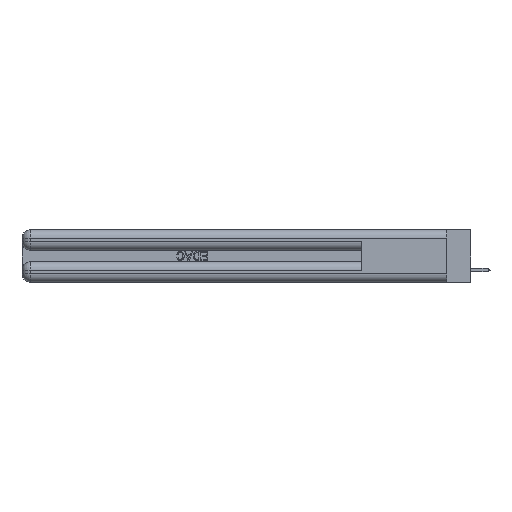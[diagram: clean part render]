
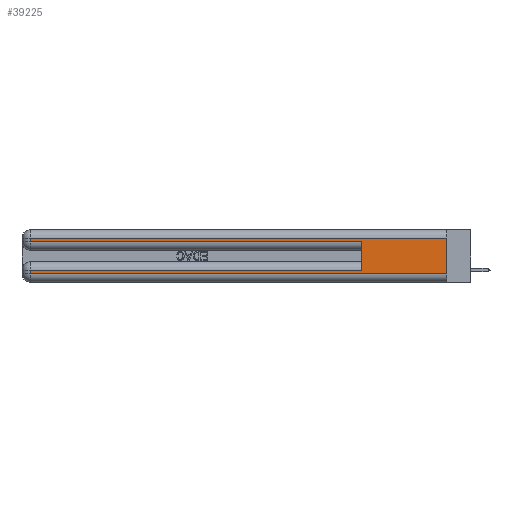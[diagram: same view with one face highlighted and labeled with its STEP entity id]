
A CAD part, left-side view. The second image highlights one B-rep face of the part: STEP entity #39225.
In plain terms, the highlighted planar face has unit normal (-1, 0, 0).
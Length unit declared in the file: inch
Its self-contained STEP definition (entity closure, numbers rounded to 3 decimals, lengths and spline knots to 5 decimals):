
#1727 = EDGE_CURVE ( 'NONE', #25122, #8568, #16309, .T. ) ;
#2623 = DIRECTION ( 'NONE',  ( 1., 0., 0. ) ) ;
#2973 = EDGE_CURVE ( 'NONE', #25122, #19299, #24184, .T. ) ;
#5003 = EDGE_CURVE ( 'NONE', #19886, #38304, #19402, .T. ) ;
#5117 = DIRECTION ( 'NONE',  ( 0., 0., -1. ) ) ;
#5318 = VECTOR ( 'NONE', #33251, 39.37008 ) ;
#7561 = LINE ( 'NONE', #8509, #25066 ) ;
#8483 = DIRECTION ( 'NONE',  ( 0., -1., 0. ) ) ;
#8509 = CARTESIAN_POINT ( 'NONE',  ( 0., 0., 0.37 ) ) ;
#8568 = VERTEX_POINT ( 'NONE', #21581 ) ;
#8902 = DIRECTION ( 'NONE',  ( 0., 0., -1. ) ) ;
#9359 = AXIS2_PLACEMENT_3D ( 'NONE', #15032, #2623, #5117 ) ;
#10208 = VECTOR ( 'NONE', #35673, 39.37008 ) ;
#10851 = CARTESIAN_POINT ( 'NONE',  ( 0., 2.94, 0.085 ) ) ;
#12128 = FACE_OUTER_BOUND ( 'NONE', #35505, .T. ) ;
#14109 = CARTESIAN_POINT ( 'NONE',  ( 0., 2.94, 0.37 ) ) ;
#14813 = LINE ( 'NONE', #34267, #28767 ) ;
#15032 = CARTESIAN_POINT ( 'NONE',  ( 0., 0., 0.37 ) ) ;
#16056 = ORIENTED_EDGE ( 'NONE', *, *, #5003, .T. ) ;
#16309 = LINE ( 'NONE', #19903, #5318 ) ;
#16492 = ORIENTED_EDGE ( 'NONE', *, *, #1727, .F. ) ;
#16751 = EDGE_CURVE ( 'NONE', #26537, #8568, #14813, .T. ) ;
#17328 = ORIENTED_EDGE ( 'NONE', *, *, #19534, .T. ) ;
#18026 = VERTEX_POINT ( 'NONE', #38992 ) ;
#18718 = ORIENTED_EDGE ( 'NONE', *, *, #16751, .T. ) ;
#19065 = LINE ( 'NONE', #14109, #24553 ) ;
#19246 = LINE ( 'NONE', #40370, #41201 ) ;
#19299 = VERTEX_POINT ( 'NONE', #10851 ) ;
#19402 = LINE ( 'NONE', #31055, #39340 ) ;
#19534 = EDGE_CURVE ( 'NONE', #25641, #26537, #19065, .T. ) ;
#19717 = DIRECTION ( 'NONE',  ( 0., 0., -1. ) ) ;
#19886 = VERTEX_POINT ( 'NONE', #36604 ) ;
#19903 = CARTESIAN_POINT ( 'NONE',  ( 0., 0.6, 0.145 ) ) ;
#20246 = DIRECTION ( 'NONE',  ( 0., 0., -1. ) ) ;
#21581 = CARTESIAN_POINT ( 'NONE',  ( 0., 0.6, 0.285 ) ) ;
#22746 = DIRECTION ( 'NONE',  ( 0., 1., 0. ) ) ;
#23398 = ORIENTED_EDGE ( 'NONE', *, *, #23899, .F. ) ;
#23899 = EDGE_CURVE ( 'NONE', #18026, #38304, #7561, .T. ) ;
#24184 = LINE ( 'NONE', #35378, #34629 ) ;
#24553 = VECTOR ( 'NONE', #20246, 39.37008 ) ;
#24842 = DIRECTION ( 'NONE',  ( 0., -1., 0. ) ) ;
#25066 = VECTOR ( 'NONE', #19717, 39.37008 ) ;
#25122 = VERTEX_POINT ( 'NONE', #35357 ) ;
#25641 = VERTEX_POINT ( 'NONE', #28639 ) ;
#26537 = VERTEX_POINT ( 'NONE', #27034 ) ;
#27034 = CARTESIAN_POINT ( 'NONE',  ( 0., 2.94, 0.285 ) ) ;
#28271 = LINE ( 'NONE', #35813, #10208 ) ;
#28639 = CARTESIAN_POINT ( 'NONE',  ( 0., 2.94, 0.31 ) ) ;
#28767 = VECTOR ( 'NONE', #24842, 39.37008 ) ;
#31055 = CARTESIAN_POINT ( 'NONE',  ( 0., 0., 0.06 ) ) ;
#32611 = CARTESIAN_POINT ( 'NONE',  ( 0., 0., 0.06 ) ) ;
#33251 = DIRECTION ( 'NONE',  ( 0., 0., 1. ) ) ;
#33953 = PLANE ( 'NONE',  #9359 ) ;
#34267 = CARTESIAN_POINT ( 'NONE',  ( 0., 0., 0.285 ) ) ;
#34629 = VECTOR ( 'NONE', #22746, 39.37008 ) ;
#34935 = EDGE_CURVE ( 'NONE', #18026, #25641, #28271, .T. ) ;
#35357 = CARTESIAN_POINT ( 'NONE',  ( 0., 0.6, 0.085 ) ) ;
#35378 = CARTESIAN_POINT ( 'NONE',  ( 0., 0., 0.085 ) ) ;
#35446 = ORIENTED_EDGE ( 'NONE', *, *, #34935, .T. ) ;
#35505 = EDGE_LOOP ( 'NONE', ( #23398, #35446, #17328, #18718, #16492, #40643, #36920, #16056 ) ) ;
#35673 = DIRECTION ( 'NONE',  ( 0., 1., 0. ) ) ;
#35813 = CARTESIAN_POINT ( 'NONE',  ( 0., 0., 0.31 ) ) ;
#36443 = EDGE_CURVE ( 'NONE', #19299, #19886, #19246, .T. ) ;
#36604 = CARTESIAN_POINT ( 'NONE',  ( 0., 2.94, 0.06 ) ) ;
#36920 = ORIENTED_EDGE ( 'NONE', *, *, #36443, .T. ) ;
#38304 = VERTEX_POINT ( 'NONE', #32611 ) ;
#38992 = CARTESIAN_POINT ( 'NONE',  ( 0., 0., 0.31 ) ) ;
#39225 = ADVANCED_FACE ( 'NONE', ( #12128 ), #33953, .F. ) ;
#39340 = VECTOR ( 'NONE', #8483, 39.37008 ) ;
#40370 = CARTESIAN_POINT ( 'NONE',  ( 0., 2.94, 0.37 ) ) ;
#40643 = ORIENTED_EDGE ( 'NONE', *, *, #2973, .T. ) ;
#41201 = VECTOR ( 'NONE', #8902, 39.37008 ) ;
